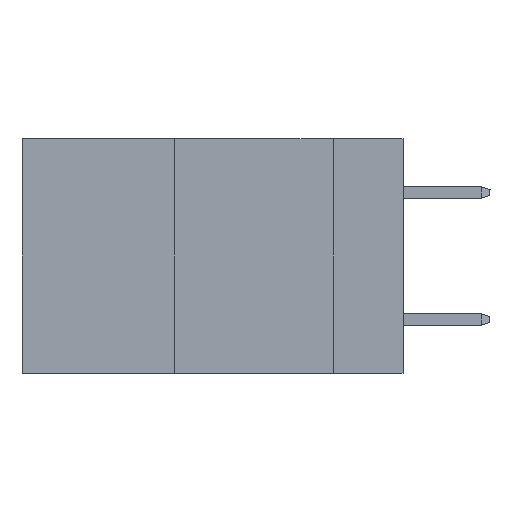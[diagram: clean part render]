
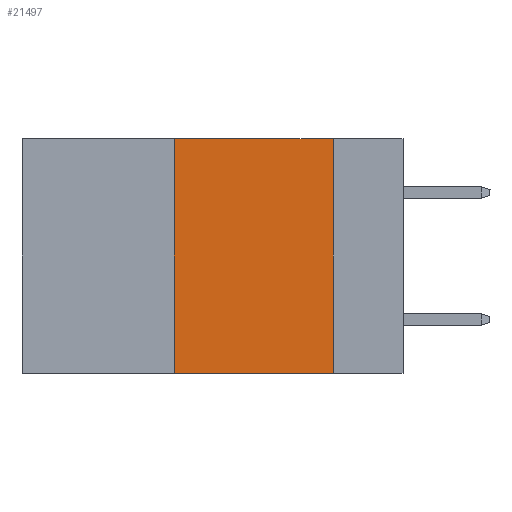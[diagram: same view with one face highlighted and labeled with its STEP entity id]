
A CAD part, left-side view. The second image highlights one B-rep face of the part: STEP entity #21497.
In plain terms, the highlighted planar face has unit normal (-1, 0, 0).
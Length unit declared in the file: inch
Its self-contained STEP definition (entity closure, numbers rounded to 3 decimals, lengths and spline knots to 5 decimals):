
#362 = PLANE ( 'NONE',  #24296 ) ;
#2492 = CARTESIAN_POINT ( 'NONE',  ( 0., 0.11, 0. ) ) ;
#3554 = CARTESIAN_POINT ( 'NONE',  ( 0., 0.6, 0. ) ) ;
#3703 = VERTEX_POINT ( 'NONE', #7417 ) ;
#5819 = CARTESIAN_POINT ( 'NONE',  ( 0., 0.6, -0.37 ) ) ;
#6453 = DIRECTION ( 'NONE',  ( 0., 0., -1. ) ) ;
#7417 = CARTESIAN_POINT ( 'NONE',  ( 0., 0.36, -0.37 ) ) ;
#7702 = ORIENTED_EDGE ( 'NONE', *, *, #38246, .T. ) ;
#9606 = EDGE_LOOP ( 'NONE', ( #30822, #36121, #17560, #7702 ) ) ;
#10509 = DIRECTION ( 'NONE',  ( 0., 0., -1. ) ) ;
#12326 = EDGE_CURVE ( 'NONE', #3703, #14818, #24411, .T. ) ;
#13069 = LINE ( 'NONE', #5819, #42550 ) ;
#13270 = LINE ( 'NONE', #3554, #21576 ) ;
#13807 = DIRECTION ( 'NONE',  ( 1., 0., 0. ) ) ;
#14007 = CARTESIAN_POINT ( 'NONE',  ( 0., 0.36, 0. ) ) ;
#14483 = EDGE_CURVE ( 'NONE', #14818, #26601, #13270, .T. ) ;
#14818 = VERTEX_POINT ( 'NONE', #29379 ) ;
#17436 = DIRECTION ( 'NONE',  ( 0., -1., 0. ) ) ;
#17536 = VERTEX_POINT ( 'NONE', #42752 ) ;
#17560 = ORIENTED_EDGE ( 'NONE', *, *, #12326, .F. ) ;
#21497 = ADVANCED_FACE ( 'NONE', ( #27537 ), #362, .F. ) ;
#21576 = VECTOR ( 'NONE', #17436, 39.37008 ) ;
#23694 = EDGE_CURVE ( 'NONE', #26601, #17536, #30092, .T. ) ;
#24213 = CARTESIAN_POINT ( 'NONE',  ( 0., 0.6, 0. ) ) ;
#24296 = AXIS2_PLACEMENT_3D ( 'NONE', #24213, #13807, #10509 ) ;
#24411 = LINE ( 'NONE', #14007, #35416 ) ;
#26601 = VERTEX_POINT ( 'NONE', #38087 ) ;
#27537 = FACE_OUTER_BOUND ( 'NONE', #9606, .T. ) ;
#29205 = VECTOR ( 'NONE', #6453, 39.37008 ) ;
#29379 = CARTESIAN_POINT ( 'NONE',  ( 0., 0.36, 0. ) ) ;
#30092 = LINE ( 'NONE', #2492, #29205 ) ;
#30822 = ORIENTED_EDGE ( 'NONE', *, *, #23694, .F. ) ;
#35416 = VECTOR ( 'NONE', #41377, 39.37008 ) ;
#36084 = DIRECTION ( 'NONE',  ( 0., -1., 0. ) ) ;
#36121 = ORIENTED_EDGE ( 'NONE', *, *, #14483, .F. ) ;
#38087 = CARTESIAN_POINT ( 'NONE',  ( 0., 0.11, 0. ) ) ;
#38246 = EDGE_CURVE ( 'NONE', #3703, #17536, #13069, .T. ) ;
#41377 = DIRECTION ( 'NONE',  ( 0., 0., 1. ) ) ;
#42550 = VECTOR ( 'NONE', #36084, 39.37008 ) ;
#42752 = CARTESIAN_POINT ( 'NONE',  ( 0., 0.11, -0.37 ) ) ;
